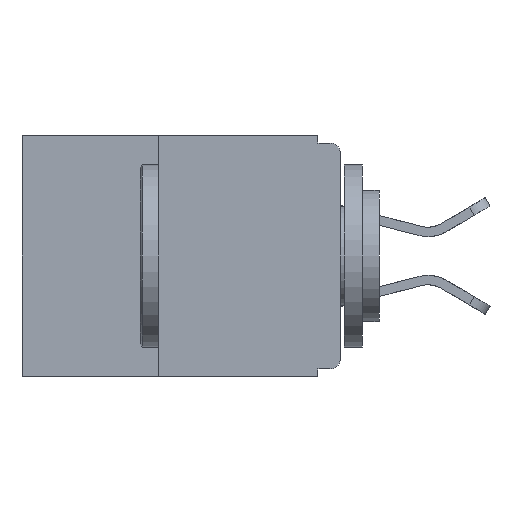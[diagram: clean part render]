
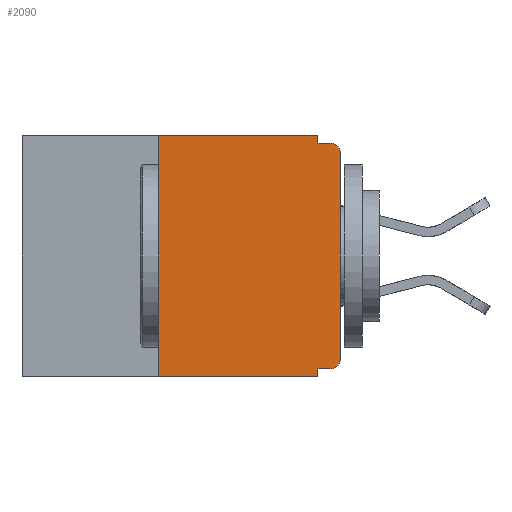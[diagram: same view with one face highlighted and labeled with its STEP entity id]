
A CAD part, left-side view. The second image highlights one B-rep face of the part: STEP entity #2090.
In plain terms, the highlighted planar face has unit normal (-1, 0, 0).
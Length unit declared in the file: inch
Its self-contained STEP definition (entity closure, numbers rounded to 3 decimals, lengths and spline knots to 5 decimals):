
#87 = ORIENTED_EDGE ( 'NONE', *, *, #11859, .T. ) ;
#147 = EDGE_CURVE ( 'NONE', #17592, #8463, #4100, .T. ) ;
#176 = CARTESIAN_POINT ( 'NONE',  ( 0., 0., -0.01 ) ) ;
#393 = DIRECTION ( 'NONE',  ( 0., 0., 1. ) ) ;
#441 = CARTESIAN_POINT ( 'NONE',  ( 0., 0., 0. ) ) ;
#1486 = VERTEX_POINT ( 'NONE', #11270 ) ;
#1546 = DIRECTION ( 'NONE',  ( -1., 0., 0. ) ) ;
#1812 = VECTOR ( 'NONE', #4425, 39.37008 ) ;
#1881 = EDGE_CURVE ( 'NONE', #17368, #13988, #5644, .T. ) ;
#2090 = ADVANCED_FACE ( 'NONE', ( #5870 ), #5551, .F. ) ;
#2207 = VERTEX_POINT ( 'NONE', #4912 ) ;
#2263 = AXIS2_PLACEMENT_3D ( 'NONE', #10001, #1546, #11353 ) ;
#2332 = VECTOR ( 'NONE', #15096, 39.37008 ) ;
#3134 = EDGE_CURVE ( 'NONE', #10282, #7742, #7320, .T. ) ;
#4100 = LINE ( 'NONE', #12715, #7393 ) ;
#4134 = VERTEX_POINT ( 'NONE', #8121 ) ;
#4225 = CARTESIAN_POINT ( 'NONE',  ( 0., 0.25, -0.33 ) ) ;
#4425 = DIRECTION ( 'NONE',  ( 0., -1., 0. ) ) ;
#4912 = CARTESIAN_POINT ( 'NONE',  ( 0., 0.015, -0.01 ) ) ;
#5224 = VECTOR ( 'NONE', #17484, 39.37008 ) ;
#5275 = ORIENTED_EDGE ( 'NONE', *, *, #7592, .T. ) ;
#5342 = VECTOR ( 'NONE', #14147, 39.37008 ) ;
#5446 = DIRECTION ( 'NONE',  ( 0., 0., -1. ) ) ;
#5551 = PLANE ( 'NONE',  #7612 ) ;
#5644 = LINE ( 'NONE', #17829, #1812 ) ;
#5802 = LINE ( 'NONE', #14784, #5342 ) ;
#5805 = EDGE_CURVE ( 'NONE', #10282, #1486, #6179, .T. ) ;
#5869 = EDGE_LOOP ( 'NONE', ( #5275, #87, #14983, #13533, #14172, #15641, #13154, #17349, #13639, #17158 ) ) ;
#5870 = FACE_OUTER_BOUND ( 'NONE', #5869, .T. ) ;
#5943 = CARTESIAN_POINT ( 'NONE',  ( 0., 0.031, -0.01 ) ) ;
#6179 = LINE ( 'NONE', #14623, #2332 ) ;
#6762 = CIRCLE ( 'NONE', #2263, 0.015 ) ;
#7320 = CIRCLE ( 'NONE', #13061, 0.015 ) ;
#7393 = VECTOR ( 'NONE', #13962, 39.37008 ) ;
#7592 = EDGE_CURVE ( 'NONE', #7742, #4134, #8829, .T. ) ;
#7612 = AXIS2_PLACEMENT_3D ( 'NONE', #11692, #14738, #16468 ) ;
#7742 = VERTEX_POINT ( 'NONE', #7897 ) ;
#7750 = CARTESIAN_POINT ( 'NONE',  ( 0., 0.015, -0.305 ) ) ;
#7793 = EDGE_CURVE ( 'NONE', #14830, #17592, #5802, .T. ) ;
#7897 = CARTESIAN_POINT ( 'NONE',  ( 0., 0., -0.305 ) ) ;
#8092 = CARTESIAN_POINT ( 'NONE',  ( 0., 0.031, -0.33 ) ) ;
#8121 = CARTESIAN_POINT ( 'NONE',  ( 0., 0., -0.025 ) ) ;
#8463 = VERTEX_POINT ( 'NONE', #5943 ) ;
#8524 = DIRECTION ( 'NONE',  ( 0., 0., 1. ) ) ;
#8728 = CARTESIAN_POINT ( 'NONE',  ( 0., 0.25, -0.33 ) ) ;
#8829 = LINE ( 'NONE', #441, #12060 ) ;
#8924 = LINE ( 'NONE', #8092, #5224 ) ;
#9459 = EDGE_CURVE ( 'NONE', #17368, #14830, #14307, .T. ) ;
#10001 = CARTESIAN_POINT ( 'NONE',  ( 0., 0.015, -0.025 ) ) ;
#10230 = CARTESIAN_POINT ( 'NONE',  ( 0., 0.25, 0. ) ) ;
#10282 = VERTEX_POINT ( 'NONE', #11708 ) ;
#10413 = LINE ( 'NONE', #176, #13599 ) ;
#10691 = VECTOR ( 'NONE', #8524, 39.37008 ) ;
#11270 = CARTESIAN_POINT ( 'NONE',  ( 0., 0.031, -0.32 ) ) ;
#11353 = DIRECTION ( 'NONE',  ( 0., 0., -1. ) ) ;
#11634 = EDGE_CURVE ( 'NONE', #1486, #13988, #8924, .T. ) ;
#11692 = CARTESIAN_POINT ( 'NONE',  ( 0., 0.437, 0. ) ) ;
#11708 = CARTESIAN_POINT ( 'NONE',  ( 0., 0.015, -0.32 ) ) ;
#11859 = EDGE_CURVE ( 'NONE', #4134, #2207, #6762, .T. ) ;
#12060 = VECTOR ( 'NONE', #393, 39.37008 ) ;
#12715 = CARTESIAN_POINT ( 'NONE',  ( 0., 0.031, 0. ) ) ;
#12933 = DIRECTION ( 'NONE',  ( 0., -1., 0. ) ) ;
#13061 = AXIS2_PLACEMENT_3D ( 'NONE', #7750, #14882, #5446 ) ;
#13154 = ORIENTED_EDGE ( 'NONE', *, *, #1881, .T. ) ;
#13533 = ORIENTED_EDGE ( 'NONE', *, *, #147, .F. ) ;
#13599 = VECTOR ( 'NONE', #12933, 39.37008 ) ;
#13639 = ORIENTED_EDGE ( 'NONE', *, *, #5805, .F. ) ;
#13962 = DIRECTION ( 'NONE',  ( 0., 0., -1. ) ) ;
#13988 = VERTEX_POINT ( 'NONE', #14924 ) ;
#14147 = DIRECTION ( 'NONE',  ( 0., -1., 0. ) ) ;
#14172 = ORIENTED_EDGE ( 'NONE', *, *, #7793, .F. ) ;
#14307 = LINE ( 'NONE', #8728, #10691 ) ;
#14623 = CARTESIAN_POINT ( 'NONE',  ( 0., 0., -0.32 ) ) ;
#14738 = DIRECTION ( 'NONE',  ( 1., 0., 0. ) ) ;
#14784 = CARTESIAN_POINT ( 'NONE',  ( 0., 0.437, 0. ) ) ;
#14830 = VERTEX_POINT ( 'NONE', #10230 ) ;
#14882 = DIRECTION ( 'NONE',  ( -1., 0., 0. ) ) ;
#14924 = CARTESIAN_POINT ( 'NONE',  ( 0., 0.031, -0.33 ) ) ;
#14983 = ORIENTED_EDGE ( 'NONE', *, *, #16306, .F. ) ;
#15096 = DIRECTION ( 'NONE',  ( 0., 1., 0. ) ) ;
#15641 = ORIENTED_EDGE ( 'NONE', *, *, #9459, .F. ) ;
#16306 = EDGE_CURVE ( 'NONE', #8463, #2207, #10413, .T. ) ;
#16468 = DIRECTION ( 'NONE',  ( 0., 0., -1. ) ) ;
#16998 = CARTESIAN_POINT ( 'NONE',  ( 0., 0.031, 0. ) ) ;
#17158 = ORIENTED_EDGE ( 'NONE', *, *, #3134, .T. ) ;
#17349 = ORIENTED_EDGE ( 'NONE', *, *, #11634, .F. ) ;
#17368 = VERTEX_POINT ( 'NONE', #4225 ) ;
#17484 = DIRECTION ( 'NONE',  ( 0., 0., -1. ) ) ;
#17592 = VERTEX_POINT ( 'NONE', #16998 ) ;
#17829 = CARTESIAN_POINT ( 'NONE',  ( 0., 0.437, -0.33 ) ) ;
